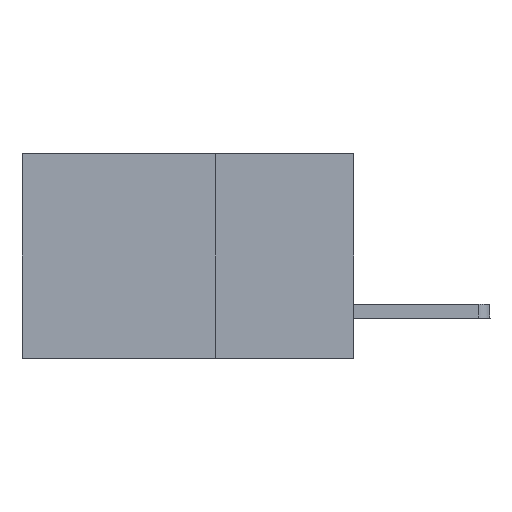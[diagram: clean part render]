
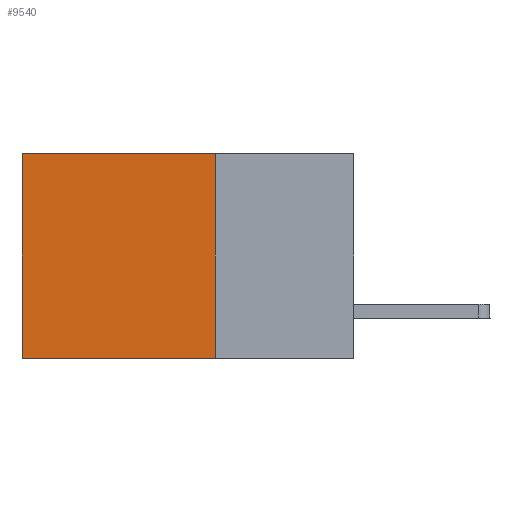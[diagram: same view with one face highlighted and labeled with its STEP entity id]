
A CAD part, left-side view. The second image highlights one B-rep face of the part: STEP entity #9540.
In plain terms, the highlighted planar face has unit normal (-1, 0, 0).
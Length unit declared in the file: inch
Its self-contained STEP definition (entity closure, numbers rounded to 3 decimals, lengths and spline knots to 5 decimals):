
#69 = CARTESIAN_POINT ( 'NONE',  ( 0.2875, 0.25, -0.37 ) ) ;
#175 = CARTESIAN_POINT ( 'NONE',  ( 0.2875, 0.25, -0.37 ) ) ;
#958 = VERTEX_POINT ( 'NONE', #69 ) ;
#1323 = VECTOR ( 'NONE', #2312, 39.37008 ) ;
#1678 = EDGE_LOOP ( 'NONE', ( #2492, #8323, #6637, #7055 ) ) ;
#2312 = DIRECTION ( 'NONE',  ( 0., 1., 0. ) ) ;
#2346 = VECTOR ( 'NONE', #9655, 39.37008 ) ;
#2492 = ORIENTED_EDGE ( 'NONE', *, *, #11728, .T. ) ;
#2691 = CARTESIAN_POINT ( 'NONE',  ( 0.2875, 0.25, 0. ) ) ;
#2893 = EDGE_CURVE ( 'NONE', #10394, #9089, #7035, .T. ) ;
#2908 = CARTESIAN_POINT ( 'NONE',  ( 0.2875, 0.6, 0. ) ) ;
#3353 = CARTESIAN_POINT ( 'NONE',  ( 0.2875, 0.25, 0. ) ) ;
#3369 = LINE ( 'NONE', #8143, #5419 ) ;
#3641 = VERTEX_POINT ( 'NONE', #5146 ) ;
#3768 = EDGE_CURVE ( 'NONE', #958, #3641, #4075, .T. ) ;
#4075 = LINE ( 'NONE', #175, #1323 ) ;
#4538 = DIRECTION ( 'NONE',  ( 0., 1., 0. ) ) ;
#4644 = DIRECTION ( 'NONE',  ( 0., 0., -1. ) ) ;
#5146 = CARTESIAN_POINT ( 'NONE',  ( 0.2875, 0.6, -0.37 ) ) ;
#5419 = VECTOR ( 'NONE', #12105, 39.37008 ) ;
#5967 = AXIS2_PLACEMENT_3D ( 'NONE', #7557, #10555, #4644 ) ;
#6637 = ORIENTED_EDGE ( 'NONE', *, *, #7975, .F. ) ;
#7035 = LINE ( 'NONE', #3353, #9364 ) ;
#7055 = ORIENTED_EDGE ( 'NONE', *, *, #2893, .T. ) ;
#7557 = CARTESIAN_POINT ( 'NONE',  ( 0.2875, 0.25, 0. ) ) ;
#7975 = EDGE_CURVE ( 'NONE', #10394, #958, #12856, .T. ) ;
#8143 = CARTESIAN_POINT ( 'NONE',  ( 0.2875, 0.6, 0. ) ) ;
#8323 = ORIENTED_EDGE ( 'NONE', *, *, #3768, .F. ) ;
#8865 = CARTESIAN_POINT ( 'NONE',  ( 0.2875, 0.25, 0. ) ) ;
#9089 = VERTEX_POINT ( 'NONE', #2908 ) ;
#9364 = VECTOR ( 'NONE', #4538, 39.37008 ) ;
#9540 = ADVANCED_FACE ( 'NONE', ( #11167 ), #9552, .F. ) ;
#9552 = PLANE ( 'NONE',  #5967 ) ;
#9655 = DIRECTION ( 'NONE',  ( 0., 0., -1. ) ) ;
#10394 = VERTEX_POINT ( 'NONE', #8865 ) ;
#10555 = DIRECTION ( 'NONE',  ( 1., 0., 0. ) ) ;
#11167 = FACE_OUTER_BOUND ( 'NONE', #1678, .T. ) ;
#11728 = EDGE_CURVE ( 'NONE', #9089, #3641, #3369, .T. ) ;
#12105 = DIRECTION ( 'NONE',  ( 0., 0., -1. ) ) ;
#12856 = LINE ( 'NONE', #2691, #2346 ) ;
